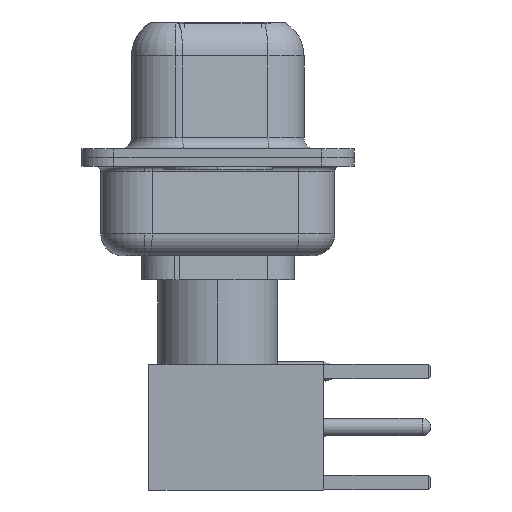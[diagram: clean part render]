
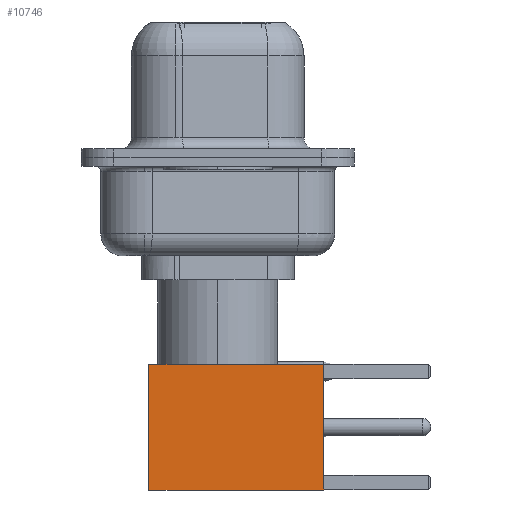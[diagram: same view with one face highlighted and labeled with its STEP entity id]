
A CAD part, left-side view. The second image highlights one B-rep face of the part: STEP entity #10746.
In plain terms, the highlighted face is planar.
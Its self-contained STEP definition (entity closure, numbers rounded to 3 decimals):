
#537 = VECTOR ( 'NONE', #23391, 1000. ) ;
#807 = ORIENTED_EDGE ( 'NONE', *, *, #19904, .F. ) ;
#1142 = CARTESIAN_POINT ( 'NONE',  ( -2.875, 2.875, 8. ) ) ;
#2466 = DIRECTION ( 'NONE',  ( -1., 0., 0. ) ) ;
#2577 = DIRECTION ( 'NONE',  ( -1., 0., 0. ) ) ;
#2691 = LINE ( 'NONE', #15552, #15478 ) ;
#4218 = DIRECTION ( 'NONE',  ( 0., 0., 1. ) ) ;
#4300 = LINE ( 'NONE', #13486, #9999 ) ;
#5484 = EDGE_CURVE ( 'NONE', #11933, #21050, #11909, .T. ) ;
#6073 = PLANE ( 'NONE',  #14888 ) ;
#8884 = CARTESIAN_POINT ( 'NONE',  ( -2.875, 2.875, 0. ) ) ;
#9489 = VERTEX_POINT ( 'NONE', #1142 ) ;
#9999 = VECTOR ( 'NONE', #2466, 1000. ) ;
#10746 = ADVANCED_FACE ( 'NONE', ( #22818 ), #6073, .T. ) ;
#10911 = ORIENTED_EDGE ( 'NONE', *, *, #14370, .F. ) ;
#11045 = CARTESIAN_POINT ( 'NONE',  ( -2.875, 2.875, 0. ) ) ;
#11909 = LINE ( 'NONE', #21427, #537 ) ;
#11933 = VERTEX_POINT ( 'NONE', #15397 ) ;
#12974 = ORIENTED_EDGE ( 'NONE', *, *, #5484, .T. ) ;
#12976 = EDGE_CURVE ( 'NONE', #21050, #15917, #4300, .T. ) ;
#13486 = CARTESIAN_POINT ( 'NONE',  ( 0., 2.875, 0. ) ) ;
#13530 = CARTESIAN_POINT ( 'NONE',  ( 2.875, 2.875, 0. ) ) ;
#14370 = EDGE_CURVE ( 'NONE', #11933, #9489, #2691, .T. ) ;
#14888 = AXIS2_PLACEMENT_3D ( 'NONE', #13530, #20978, #4218 ) ;
#15397 = CARTESIAN_POINT ( 'NONE',  ( 2.875, 2.875, 8. ) ) ;
#15478 = VECTOR ( 'NONE', #2577, 1000. ) ;
#15552 = CARTESIAN_POINT ( 'NONE',  ( 0., 2.875, 8. ) ) ;
#15917 = VERTEX_POINT ( 'NONE', #11045 ) ;
#16809 = LINE ( 'NONE', #8884, #21129 ) ;
#17598 = EDGE_LOOP ( 'NONE', ( #12974, #21521, #807, #10911 ) ) ;
#19863 = CARTESIAN_POINT ( 'NONE',  ( 2.875, 2.875, 0. ) ) ;
#19904 = EDGE_CURVE ( 'NONE', #9489, #15917, #16809, .T. ) ;
#20978 = DIRECTION ( 'NONE',  ( 0., 1., 0. ) ) ;
#21050 = VERTEX_POINT ( 'NONE', #19863 ) ;
#21129 = VECTOR ( 'NONE', #22077, 1000. ) ;
#21427 = CARTESIAN_POINT ( 'NONE',  ( 2.875, 2.875, 0. ) ) ;
#21521 = ORIENTED_EDGE ( 'NONE', *, *, #12976, .T. ) ;
#22077 = DIRECTION ( 'NONE',  ( 0., 0., -1. ) ) ;
#22818 = FACE_OUTER_BOUND ( 'NONE', #17598, .T. ) ;
#23391 = DIRECTION ( 'NONE',  ( 0., 0., -1. ) ) ;
